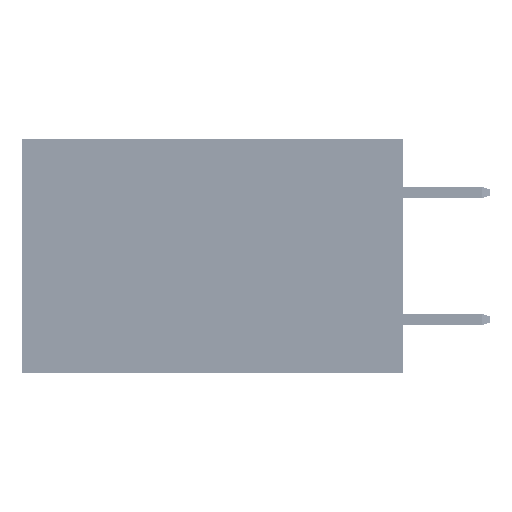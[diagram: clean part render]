
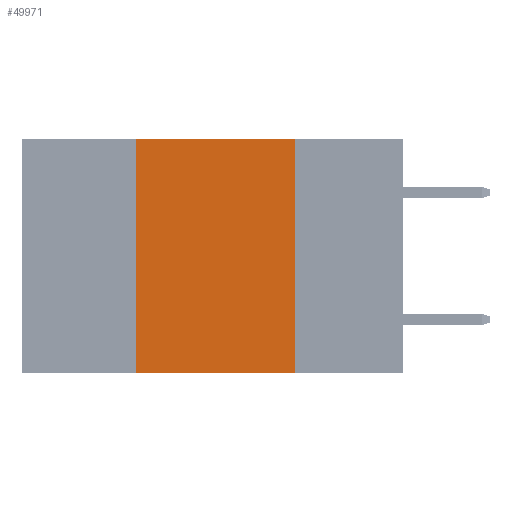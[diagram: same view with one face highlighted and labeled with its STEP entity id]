
A CAD part, left-side view. The second image highlights one B-rep face of the part: STEP entity #49971.
In plain terms, the highlighted planar face has unit normal (-1, 0, 0).
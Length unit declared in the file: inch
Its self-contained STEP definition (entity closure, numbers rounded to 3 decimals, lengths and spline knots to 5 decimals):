
#71 = ORIENTED_EDGE ( 'NONE', *, *, #34122, .T. ) ;
#729 = VECTOR ( 'NONE', #38273, 39.37008 ) ;
#4188 = EDGE_CURVE ( 'NONE', #7763, #30461, #13740, .T. ) ;
#5329 = ORIENTED_EDGE ( 'NONE', *, *, #33988, .F. ) ;
#5343 = VECTOR ( 'NONE', #21604, 39.37008 ) ;
#6516 = LINE ( 'NONE', #22785, #37601 ) ;
#7763 = VERTEX_POINT ( 'NONE', #42733 ) ;
#10338 = ORIENTED_EDGE ( 'NONE', *, *, #31288, .F. ) ;
#10621 = LINE ( 'NONE', #47183, #12127 ) ;
#11337 = VERTEX_POINT ( 'NONE', #42417 ) ;
#11973 = FACE_OUTER_BOUND ( 'NONE', #44901, .T. ) ;
#12127 = VECTOR ( 'NONE', #43162, 39.37008 ) ;
#13740 = LINE ( 'NONE', #30024, #729 ) ;
#21604 = DIRECTION ( 'NONE',  ( 0., -1., 0. ) ) ;
#22785 = CARTESIAN_POINT ( 'NONE',  ( 0., 0.42, 0. ) ) ;
#25327 = CARTESIAN_POINT ( 'NONE',  ( 0., 0.6, 0. ) ) ;
#30024 = CARTESIAN_POINT ( 'NONE',  ( 0., 0.17, 0. ) ) ;
#30461 = VERTEX_POINT ( 'NONE', #46501 ) ;
#31288 = EDGE_CURVE ( 'NONE', #11337, #47838, #6516, .T. ) ;
#33702 = CARTESIAN_POINT ( 'NONE',  ( 0., 0.42, 0. ) ) ;
#33854 = LINE ( 'NONE', #25327, #5343 ) ;
#33967 = ORIENTED_EDGE ( 'NONE', *, *, #4188, .F. ) ;
#33988 = EDGE_CURVE ( 'NONE', #47838, #7763, #33854, .T. ) ;
#34122 = EDGE_CURVE ( 'NONE', #11337, #30461, #10621, .T. ) ;
#35201 = DIRECTION ( 'NONE',  ( 0., 0., -1. ) ) ;
#37601 = VECTOR ( 'NONE', #39057, 39.37008 ) ;
#38273 = DIRECTION ( 'NONE',  ( 0., 0., -1. ) ) ;
#39057 = DIRECTION ( 'NONE',  ( 0., 0., 1. ) ) ;
#42417 = CARTESIAN_POINT ( 'NONE',  ( 0., 0.42, -0.37 ) ) ;
#42733 = CARTESIAN_POINT ( 'NONE',  ( 0., 0.17, 0. ) ) ;
#43162 = DIRECTION ( 'NONE',  ( 0., -1., 0. ) ) ;
#43749 = PLANE ( 'NONE',  #48495 ) ;
#44901 = EDGE_LOOP ( 'NONE', ( #33967, #5329, #10338, #71 ) ) ;
#46501 = CARTESIAN_POINT ( 'NONE',  ( 0., 0.17, -0.37 ) ) ;
#47183 = CARTESIAN_POINT ( 'NONE',  ( 0., 0.6, -0.37 ) ) ;
#47838 = VERTEX_POINT ( 'NONE', #33702 ) ;
#48027 = DIRECTION ( 'NONE',  ( 1., 0., 0. ) ) ;
#48495 = AXIS2_PLACEMENT_3D ( 'NONE', #51752, #48027, #35201 ) ;
#49971 = ADVANCED_FACE ( 'NONE', ( #11973 ), #43749, .F. ) ;
#51752 = CARTESIAN_POINT ( 'NONE',  ( 0., 0.6, 0. ) ) ;
